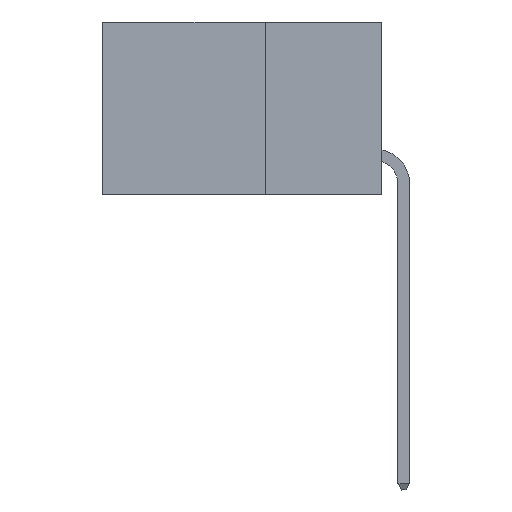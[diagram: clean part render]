
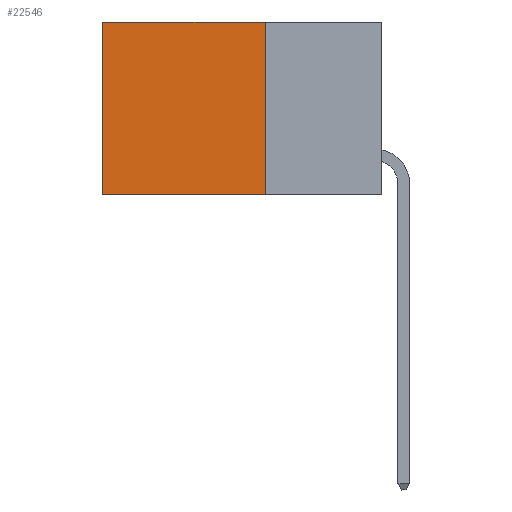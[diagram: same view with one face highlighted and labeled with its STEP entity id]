
A CAD part, left-side view. The second image highlights one B-rep face of the part: STEP entity #22546.
In plain terms, the highlighted planar face has unit normal (-1, 0, 0).
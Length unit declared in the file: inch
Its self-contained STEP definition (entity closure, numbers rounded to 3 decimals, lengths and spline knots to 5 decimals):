
#748 = CARTESIAN_POINT ( 'NONE',  ( 0.2875, 0.6, -0.37 ) ) ;
#3051 = LINE ( 'NONE', #19916, #27729 ) ;
#4046 = CARTESIAN_POINT ( 'NONE',  ( 0.2875, 0.25, -0.37 ) ) ;
#5236 = EDGE_CURVE ( 'NONE', #15108, #10526, #10719, .T. ) ;
#5397 = CARTESIAN_POINT ( 'NONE',  ( 0.2875, 0.25, 0. ) ) ;
#6065 = EDGE_CURVE ( 'NONE', #10526, #18998, #25934, .T. ) ;
#9755 = DIRECTION ( 'NONE',  ( 0., 1., 0. ) ) ;
#10526 = VERTEX_POINT ( 'NONE', #4046 ) ;
#10719 = LINE ( 'NONE', #36896, #16503 ) ;
#11132 = DIRECTION ( 'NONE',  ( 0., 0., -1. ) ) ;
#11346 = EDGE_LOOP ( 'NONE', ( #13069, #19406, #15059, #21104 ) ) ;
#13069 = ORIENTED_EDGE ( 'NONE', *, *, #32629, .T. ) ;
#13654 = AXIS2_PLACEMENT_3D ( 'NONE', #5397, #37175, #11132 ) ;
#13840 = DIRECTION ( 'NONE',  ( 0., 0., -1. ) ) ;
#15059 = ORIENTED_EDGE ( 'NONE', *, *, #5236, .F. ) ;
#15108 = VERTEX_POINT ( 'NONE', #27334 ) ;
#15372 = LINE ( 'NONE', #37014, #21216 ) ;
#16503 = VECTOR ( 'NONE', #13840, 39.37008 ) ;
#18998 = VERTEX_POINT ( 'NONE', #748 ) ;
#19406 = ORIENTED_EDGE ( 'NONE', *, *, #6065, .F. ) ;
#19743 = CARTESIAN_POINT ( 'NONE',  ( 0.2875, 0.6, 0. ) ) ;
#19916 = CARTESIAN_POINT ( 'NONE',  ( 0.2875, 0.6, 0. ) ) ;
#20205 = FACE_OUTER_BOUND ( 'NONE', #11346, .T. ) ;
#21104 = ORIENTED_EDGE ( 'NONE', *, *, #21347, .T. ) ;
#21216 = VECTOR ( 'NONE', #31590, 39.37008 ) ;
#21303 = CARTESIAN_POINT ( 'NONE',  ( 0.2875, 0.25, -0.37 ) ) ;
#21347 = EDGE_CURVE ( 'NONE', #15108, #25144, #15372, .T. ) ;
#22546 = ADVANCED_FACE ( 'NONE', ( #20205 ), #31368, .F. ) ;
#25144 = VERTEX_POINT ( 'NONE', #19743 ) ;
#25934 = LINE ( 'NONE', #21303, #30898 ) ;
#27334 = CARTESIAN_POINT ( 'NONE',  ( 0.2875, 0.25, 0. ) ) ;
#27729 = VECTOR ( 'NONE', #37065, 39.37008 ) ;
#30898 = VECTOR ( 'NONE', #9755, 39.37008 ) ;
#31368 = PLANE ( 'NONE',  #13654 ) ;
#31590 = DIRECTION ( 'NONE',  ( 0., 1., 0. ) ) ;
#32629 = EDGE_CURVE ( 'NONE', #25144, #18998, #3051, .T. ) ;
#36896 = CARTESIAN_POINT ( 'NONE',  ( 0.2875, 0.25, 0. ) ) ;
#37014 = CARTESIAN_POINT ( 'NONE',  ( 0.2875, 0.25, 0. ) ) ;
#37065 = DIRECTION ( 'NONE',  ( 0., 0., -1. ) ) ;
#37175 = DIRECTION ( 'NONE',  ( 1., 0., 0. ) ) ;
